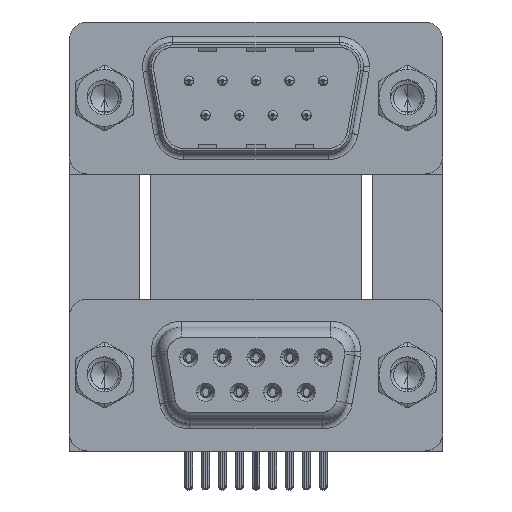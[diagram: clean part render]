
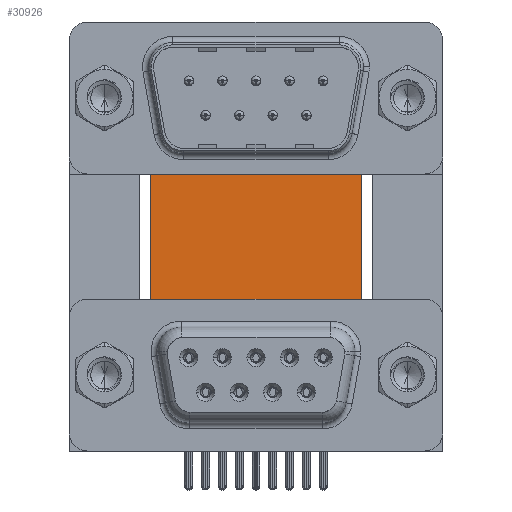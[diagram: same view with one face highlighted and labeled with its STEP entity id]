
A CAD part, top view. The second image highlights one B-rep face of the part: STEP entity #30926.
In plain terms, the highlighted planar face has unit normal (0, 0, 1).
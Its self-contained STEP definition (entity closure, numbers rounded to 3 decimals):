
#112 = VERTEX_POINT ( 'NONE', #19013 ) ;
#129 = CARTESIAN_POINT ( 'NONE',  ( 22.59, -4.635, -12. ) ) ;
#2044 = VERTEX_POINT ( 'NONE', #18163 ) ;
#2749 = ORIENTED_EDGE ( 'NONE', *, *, #33802, .F. ) ;
#3138 = ORIENTED_EDGE ( 'NONE', *, *, #27010, .T. ) ;
#3176 = DIRECTION ( 'NONE',  ( 1., 0., 0. ) ) ;
#3177 = VECTOR ( 'NONE', #42182, 1000. ) ;
#3267 = VECTOR ( 'NONE', #40461, 1000. ) ;
#4741 = LINE ( 'NONE', #15108, #12782 ) ;
#4854 = VERTEX_POINT ( 'NONE', #30442 ) ;
#4857 = LINE ( 'NONE', #32998, #28680 ) ;
#4950 = VECTOR ( 'NONE', #24209, 1000. ) ;
#5106 = DIRECTION ( 'NONE',  ( 1., 0., 0. ) ) ;
#5912 = CARTESIAN_POINT ( 'NONE',  ( 3.79, -0.735, -12. ) ) ;
#6656 = CARTESIAN_POINT ( 'NONE',  ( 3.79, 16.585, -12. ) ) ;
#6677 = CARTESIAN_POINT ( 'NONE',  ( 22.09, -4.635, -12. ) ) ;
#7268 = LINE ( 'NONE', #20982, #37031 ) ;
#7350 = LINE ( 'NONE', #129, #4950 ) ;
#7425 = VECTOR ( 'NONE', #14882, 1000. ) ;
#8492 = LINE ( 'NONE', #22214, #42382 ) ;
#8810 = ORIENTED_EDGE ( 'NONE', *, *, #44097, .T. ) ;
#9141 = DIRECTION ( 'NONE',  ( 0., -1., 0. ) ) ;
#10288 = CARTESIAN_POINT ( 'NONE',  ( 22.09, -3.735, -12. ) ) ;
#10855 = EDGE_CURVE ( 'NONE', #36632, #24624, #38535, .T. ) ;
#12535 = CARTESIAN_POINT ( 'NONE',  ( 21.2, 16.585, -12. ) ) ;
#12782 = VECTOR ( 'NONE', #32874, 1000. ) ;
#12891 = VERTEX_POINT ( 'NONE', #5912 ) ;
#13255 = PLANE ( 'NONE',  #32120 ) ;
#13466 = EDGE_CURVE ( 'NONE', #20601, #4854, #7268, .T. ) ;
#14471 = ORIENTED_EDGE ( 'NONE', *, *, #10855, .T. ) ;
#14882 = DIRECTION ( 'NONE',  ( 1., 0., 0. ) ) ;
#15108 = CARTESIAN_POINT ( 'NONE',  ( 3.79, 16.585, -12. ) ) ;
#15244 = ORIENTED_EDGE ( 'NONE', *, *, #42976, .T. ) ;
#15982 = FACE_OUTER_BOUND ( 'NONE', #43308, .T. ) ;
#16458 = VECTOR ( 'NONE', #23298, 1000. ) ;
#17947 = VERTEX_POINT ( 'NONE', #43999 ) ;
#18077 = LINE ( 'NONE', #39240, #3177 ) ;
#18163 = CARTESIAN_POINT ( 'NONE',  ( 2.9, -4.635, -12. ) ) ;
#19013 = CARTESIAN_POINT ( 'NONE',  ( 3.79, 16.585, -12. ) ) ;
#20601 = VERTEX_POINT ( 'NONE', #6677 ) ;
#20778 = EDGE_CURVE ( 'NONE', #4854, #33558, #7350, .T. ) ;
#20982 = CARTESIAN_POINT ( 'NONE',  ( 22.09, -4.635, -12. ) ) ;
#21443 = VECTOR ( 'NONE', #25878, 1000. ) ;
#21894 = ORIENTED_EDGE ( 'NONE', *, *, #25198, .T. ) ;
#22214 = CARTESIAN_POINT ( 'NONE',  ( 2.9, -4.635, -12. ) ) ;
#22595 = CARTESIAN_POINT ( 'NONE',  ( 2.9, -3.735, -12. ) ) ;
#23298 = DIRECTION ( 'NONE',  ( 1., 0., 0. ) ) ;
#24209 = DIRECTION ( 'NONE',  ( -0.336, 0.942, 0. ) ) ;
#24624 = VERTEX_POINT ( 'NONE', #32657 ) ;
#25123 = CARTESIAN_POINT ( 'NONE',  ( 21.2, -0.735, -12. ) ) ;
#25198 = EDGE_CURVE ( 'NONE', #12891, #17947, #18077, .T. ) ;
#25878 = DIRECTION ( 'NONE',  ( 0., 1., 0. ) ) ;
#26956 = DIRECTION ( 'NONE',  ( 0., 0., -1. ) ) ;
#27010 = EDGE_CURVE ( 'NONE', #24624, #20601, #44297, .T. ) ;
#28680 = VECTOR ( 'NONE', #9141, 1000. ) ;
#30343 = LINE ( 'NONE', #36703, #21443 ) ;
#30442 = CARTESIAN_POINT ( 'NONE',  ( 22.59, -4.635, -12. ) ) ;
#30926 = ADVANCED_FACE ( 'NONE', ( #15982 ), #13255, .F. ) ;
#32120 = AXIS2_PLACEMENT_3D ( 'NONE', #36902, #26956, #37344 ) ;
#32657 = CARTESIAN_POINT ( 'NONE',  ( 22.09, -3.735, -12. ) ) ;
#32874 = DIRECTION ( 'NONE',  ( 0., -1., 0. ) ) ;
#32998 = CARTESIAN_POINT ( 'NONE',  ( 21.2, 16.585, -12. ) ) ;
#33237 = LINE ( 'NONE', #6656, #16458 ) ;
#33558 = VERTEX_POINT ( 'NONE', #25123 ) ;
#33802 = EDGE_CURVE ( 'NONE', #36101, #33558, #4857, .T. ) ;
#35126 = EDGE_CURVE ( 'NONE', #112, #36101, #33237, .T. ) ;
#36101 = VERTEX_POINT ( 'NONE', #12535 ) ;
#36183 = EDGE_CURVE ( 'NONE', #17947, #2044, #8492, .T. ) ;
#36632 = VERTEX_POINT ( 'NONE', #22595 ) ;
#36703 = CARTESIAN_POINT ( 'NONE',  ( 2.9, -3.735, -12. ) ) ;
#36902 = CARTESIAN_POINT ( 'NONE',  ( 3.79, 16.585, -12. ) ) ;
#37031 = VECTOR ( 'NONE', #3176, 1000. ) ;
#37344 = DIRECTION ( 'NONE',  ( -1., 0., 0. ) ) ;
#37844 = ORIENTED_EDGE ( 'NONE', *, *, #13466, .T. ) ;
#38291 = ORIENTED_EDGE ( 'NONE', *, *, #36183, .T. ) ;
#38535 = LINE ( 'NONE', #41924, #7425 ) ;
#38910 = ORIENTED_EDGE ( 'NONE', *, *, #20778, .T. ) ;
#39214 = ORIENTED_EDGE ( 'NONE', *, *, #35126, .F. ) ;
#39240 = CARTESIAN_POINT ( 'NONE',  ( 2.4, -4.635, -12. ) ) ;
#40461 = DIRECTION ( 'NONE',  ( 0., -1., 0. ) ) ;
#41924 = CARTESIAN_POINT ( 'NONE',  ( 3.79, -3.735, -12. ) ) ;
#42182 = DIRECTION ( 'NONE',  ( -0.336, -0.942, 0. ) ) ;
#42382 = VECTOR ( 'NONE', #5106, 1000. ) ;
#42976 = EDGE_CURVE ( 'NONE', #2044, #36632, #30343, .T. ) ;
#43308 = EDGE_LOOP ( 'NONE', ( #14471, #3138, #37844, #38910, #2749, #39214, #8810, #21894, #38291, #15244 ) ) ;
#43999 = CARTESIAN_POINT ( 'NONE',  ( 2.4, -4.635, -12. ) ) ;
#44097 = EDGE_CURVE ( 'NONE', #112, #12891, #4741, .T. ) ;
#44297 = LINE ( 'NONE', #10288, #3267 ) ;
